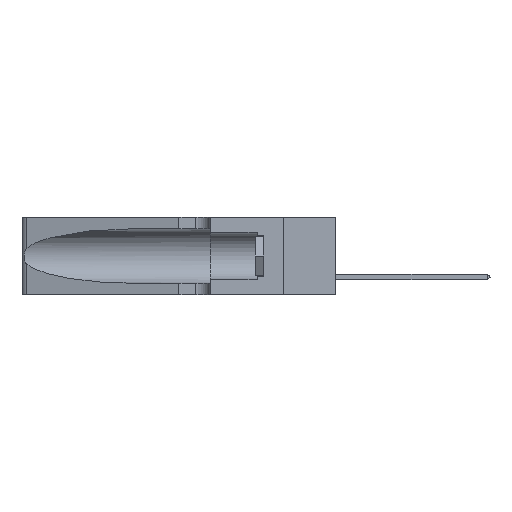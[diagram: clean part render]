
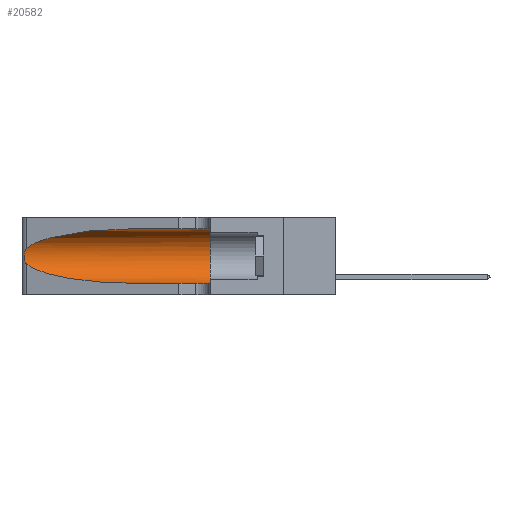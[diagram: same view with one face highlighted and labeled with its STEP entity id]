
A CAD part, left-side view. The second image highlights one B-rep face of the part: STEP entity #20582.
In plain terms, the highlighted cylindrical face has radius 3.308 mm (diameter 6.617 mm), a partial arc.
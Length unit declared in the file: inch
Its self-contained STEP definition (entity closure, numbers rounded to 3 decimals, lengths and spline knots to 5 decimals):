
#113 = CARTESIAN_POINT ( 'NONE',  ( 0.25555, 1.22993, 0.14849 ) ) ;
#267 = EDGE_CURVE ( 'NONE', #17366, #27571, #12175, .T. ) ;
#426 = CARTESIAN_POINT ( 'NONE',  ( 0.18966, 0.96281, 0.05475 ) ) ;
#996 = EDGE_CURVE ( 'NONE', #6347, #10217, #15327, .T. ) ;
#2148 = ORIENTED_EDGE ( 'NONE', *, *, #267, .T. ) ;
#2304 = DIRECTION ( 'NONE',  ( 0., -1., 0. ) ) ;
#2311 = CARTESIAN_POINT ( 'NONE',  ( 0.25555, 1.22994, 0.2215 ) ) ;
#2392 = CARTESIAN_POINT ( 'NONE',  ( 0.1305, 0.72297, 0.31525 ) ) ;
#2410 = CARTESIAN_POINT ( 'NONE',  ( 0.25487, 1.22718, 0.14631 ) ) ;
#2477 = VECTOR ( 'NONE', #11126, 39.37008 ) ;
#2488 = EDGE_CURVE ( 'NONE', #12129, #9983, #11263, .T. ) ;
#3360 = EDGE_LOOP ( 'NONE', ( #23242, #28286, #22555, #2148, #9365, #18984 ) ) ;
#4528 = CARTESIAN_POINT ( 'NONE',  ( 0.26075, 1.23896, 0.19203 ) ) ;
#4628 = CARTESIAN_POINT ( 'NONE',  ( 0.25856, 1.23593, 0.16098 ) ) ;
#6347 = VERTEX_POINT ( 'NONE', #26857 ) ;
#6818 = CARTESIAN_POINT ( 'NONE',  ( 0.1305, 0.35, 0.185 ) ) ;
#6836 = CARTESIAN_POINT ( 'NONE',  ( 0.25487, 1.22718, 0.22369 ) ) ;
#8692 =( BOUNDED_CURVE ( )  B_SPLINE_CURVE ( 3, ( #2392, #9099, #22554, #24807 ),
 .UNSPECIFIED., .F., .F. ) 
 B_SPLINE_CURVE_WITH_KNOTS ( ( 4, 4 ),
 ( 1.5708, 2.84003 ),
 .UNSPECIFIED. ) 
 CURVE ( )  GEOMETRIC_REPRESENTATION_ITEM ( )  RATIONAL_B_SPLINE_CURVE ( ( 1., 0.87, 0.87, 1. ) ) 
 REPRESENTATION_ITEM ( '' )  );
#9099 = CARTESIAN_POINT ( 'NONE',  ( 0.18966, 0.96281, 0.31525 ) ) ;
#9197 = DIRECTION ( 'NONE',  ( 0., 0., 1. ) ) ;
#9309 = CARTESIAN_POINT ( 'NONE',  ( 0.26018, 1.23835, 0.19895 ) ) ;
#9342 = CARTESIAN_POINT ( 'NONE',  ( 0.1305, 0.72297, 0.05475 ) ) ;
#9365 = ORIENTED_EDGE ( 'NONE', *, *, #22429, .F. ) ;
#9983 = VERTEX_POINT ( 'NONE', #13367 ) ;
#10217 = VERTEX_POINT ( 'NONE', #25220 ) ;
#10384 = VECTOR ( 'NONE', #2304, 39.37008 ) ;
#11126 = DIRECTION ( 'NONE',  ( 0., -1., 0. ) ) ;
#11263 = B_SPLINE_CURVE_WITH_KNOTS ( 'NONE', 3,
 ( #25089, #2311, #18265, #11420, #29369, #9309, #4528, #11599, #18463, #4628, #11313, #27460, #113, #2410 ),
 .UNSPECIFIED., .F., .F.,
 ( 4, 2, 2, 2, 2, 2, 4 ),
 ( 0., 0.00027, 0.00053, 0.00107, 0.0016, 0.00187, 0.00214 ),
 .UNSPECIFIED. ) ;
#11313 = CARTESIAN_POINT ( 'NONE',  ( 0.25789, 1.23486, 0.15765 ) ) ;
#11420 = CARTESIAN_POINT ( 'NONE',  ( 0.25787, 1.23484, 0.2124 ) ) ;
#11599 = CARTESIAN_POINT ( 'NONE',  ( 0.26075, 1.23896, 0.178 ) ) ;
#12129 = VERTEX_POINT ( 'NONE', #6836 ) ;
#12175 = LINE ( 'NONE', #13974, #10384 ) ;
#12321 = CARTESIAN_POINT ( 'NONE',  ( 0.1305, 1.61858, 0.185 ) ) ;
#13367 = CARTESIAN_POINT ( 'NONE',  ( 0.25487, 1.22718, 0.14631 ) ) ;
#13386 = DIRECTION ( 'NONE',  ( 0., 1., 0. ) ) ;
#13974 = CARTESIAN_POINT ( 'NONE',  ( 0.1305, 1.61858, 0.05475 ) ) ;
#15327 = LINE ( 'NONE', #16106, #2477 ) ;
#16106 = CARTESIAN_POINT ( 'NONE',  ( 0.1305, 1.61858, 0.31525 ) ) ;
#17004 = DIRECTION ( 'NONE',  ( 0., 0., -1. ) ) ;
#17366 = VERTEX_POINT ( 'NONE', #25727 ) ;
#17722 = AXIS2_PLACEMENT_3D ( 'NONE', #12321, #19300, #17004 ) ;
#17910 = CARTESIAN_POINT ( 'NONE',  ( 0.1305, 0.35, 0.05475 ) ) ;
#18265 = CARTESIAN_POINT ( 'NONE',  ( 0.25639, 1.23184, 0.21858 ) ) ;
#18463 = CARTESIAN_POINT ( 'NONE',  ( 0.26017, 1.23833, 0.17102 ) ) ;
#18984 = ORIENTED_EDGE ( 'NONE', *, *, #996, .F. ) ;
#19300 = DIRECTION ( 'NONE',  ( 0., -1., 0. ) ) ;
#20582 = ADVANCED_FACE ( 'NONE', ( #23682 ), #22986, .F. ) ;
#21116 =( BOUNDED_CURVE ( )  B_SPLINE_CURVE ( 3, ( #23077, #25410, #426, #9342 ),
 .UNSPECIFIED., .F., .F. ) 
 B_SPLINE_CURVE_WITH_KNOTS ( ( 4, 4 ),
 ( 3.44316, 4.71239 ),
 .UNSPECIFIED. ) 
 CURVE ( )  GEOMETRIC_REPRESENTATION_ITEM ( )  RATIONAL_B_SPLINE_CURVE ( ( 1., 0.87, 0.87, 1. ) ) 
 REPRESENTATION_ITEM ( '' )  );
#21232 = AXIS2_PLACEMENT_3D ( 'NONE', #6818, #13386, #9197 ) ;
#22429 = EDGE_CURVE ( 'NONE', #10217, #27571, #25022, .T. ) ;
#22554 = CARTESIAN_POINT ( 'NONE',  ( 0.2373, 1.15595, 0.28018 ) ) ;
#22555 = ORIENTED_EDGE ( 'NONE', *, *, #26189, .T. ) ;
#22986 = CYLINDRICAL_SURFACE ( 'NONE', #17722, 0.13025 ) ;
#23077 = CARTESIAN_POINT ( 'NONE',  ( 0.25487, 1.22718, 0.14631 ) ) ;
#23242 = ORIENTED_EDGE ( 'NONE', *, *, #23656, .T. ) ;
#23656 = EDGE_CURVE ( 'NONE', #6347, #12129, #8692, .T. ) ;
#23682 = FACE_OUTER_BOUND ( 'NONE', #3360, .T. ) ;
#24807 = CARTESIAN_POINT ( 'NONE',  ( 0.25487, 1.22718, 0.22369 ) ) ;
#25022 = CIRCLE ( 'NONE', #21232, 0.13025 ) ;
#25089 = CARTESIAN_POINT ( 'NONE',  ( 0.25487, 1.22718, 0.22369 ) ) ;
#25220 = CARTESIAN_POINT ( 'NONE',  ( 0.1305, 0.35, 0.31525 ) ) ;
#25410 = CARTESIAN_POINT ( 'NONE',  ( 0.2373, 1.15595, 0.08982 ) ) ;
#25727 = CARTESIAN_POINT ( 'NONE',  ( 0.1305, 0.72297, 0.05475 ) ) ;
#26189 = EDGE_CURVE ( 'NONE', #9983, #17366, #21116, .T. ) ;
#26857 = CARTESIAN_POINT ( 'NONE',  ( 0.1305, 0.72297, 0.31525 ) ) ;
#27460 = CARTESIAN_POINT ( 'NONE',  ( 0.25639, 1.23186, 0.15144 ) ) ;
#27571 = VERTEX_POINT ( 'NONE', #17910 ) ;
#28286 = ORIENTED_EDGE ( 'NONE', *, *, #2488, .T. ) ;
#29369 = CARTESIAN_POINT ( 'NONE',  ( 0.25854, 1.2359, 0.20912 ) ) ;
